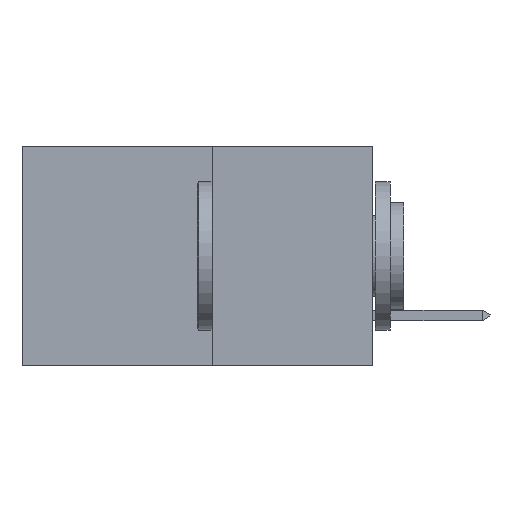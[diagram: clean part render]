
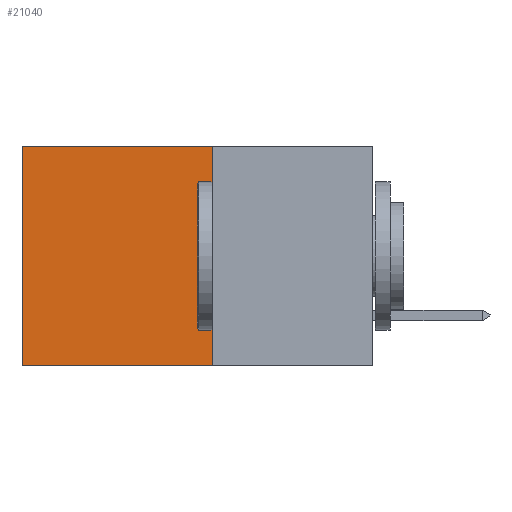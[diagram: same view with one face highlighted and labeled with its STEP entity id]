
A CAD part, left-side view. The second image highlights one B-rep face of the part: STEP entity #21040.
In plain terms, the highlighted planar face has unit normal (-1, 0, 0).
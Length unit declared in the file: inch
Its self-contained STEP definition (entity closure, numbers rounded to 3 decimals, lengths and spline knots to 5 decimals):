
#260 = DIRECTION ( 'NONE',  ( 0., 0., -1. ) ) ;
#1293 = LINE ( 'NONE', #17203, #12960 ) ;
#1573 = PLANE ( 'NONE',  #18621 ) ;
#2381 = EDGE_CURVE ( 'NONE', #3622, #14058, #3923, .T. ) ;
#2585 = CARTESIAN_POINT ( 'NONE',  ( 0.277, 0.27, 0. ) ) ;
#3622 = VERTEX_POINT ( 'NONE', #2585 ) ;
#3923 = LINE ( 'NONE', #11362, #9399 ) ;
#4416 = CARTESIAN_POINT ( 'NONE',  ( 0.277, 0.59, -0.37 ) ) ;
#6272 = DIRECTION ( 'NONE',  ( 0., 0., -1. ) ) ;
#6771 = DIRECTION ( 'NONE',  ( 0., 0., -1. ) ) ;
#6884 = CARTESIAN_POINT ( 'NONE',  ( 0.277, 0.59, 0. ) ) ;
#7058 = ORIENTED_EDGE ( 'NONE', *, *, #27936, .F. ) ;
#7704 = LINE ( 'NONE', #4416, #19350 ) ;
#9399 = VECTOR ( 'NONE', #25310, 39.37008 ) ;
#11069 = CARTESIAN_POINT ( 'NONE',  ( 0.277, 0.59, -0.37 ) ) ;
#11362 = CARTESIAN_POINT ( 'NONE',  ( 0.277, 0.27, 0. ) ) ;
#12960 = VECTOR ( 'NONE', #19562, 39.37008 ) ;
#14058 = VERTEX_POINT ( 'NONE', #6884 ) ;
#17203 = CARTESIAN_POINT ( 'NONE',  ( 0.277, 0.27, -0.37 ) ) ;
#17643 = CARTESIAN_POINT ( 'NONE',  ( 0.277, 0.27, -0.37 ) ) ;
#17770 = VERTEX_POINT ( 'NONE', #11069 ) ;
#17841 = CARTESIAN_POINT ( 'NONE',  ( 0.277, 0.27, -0.37 ) ) ;
#17953 = FACE_OUTER_BOUND ( 'NONE', #29388, .T. ) ;
#18621 = AXIS2_PLACEMENT_3D ( 'NONE', #17841, #20214, #6272 ) ;
#18826 = ORIENTED_EDGE ( 'NONE', *, *, #23870, .T. ) ;
#19350 = VECTOR ( 'NONE', #6771, 39.37008 ) ;
#19562 = DIRECTION ( 'NONE',  ( 0., 1., 0. ) ) ;
#20214 = DIRECTION ( 'NONE',  ( 1., 0., 0. ) ) ;
#20658 = VECTOR ( 'NONE', #260, 39.37008 ) ;
#20684 = ORIENTED_EDGE ( 'NONE', *, *, #27000, .F. ) ;
#21040 = ADVANCED_FACE ( 'NONE', ( #17953 ), #1573, .F. ) ;
#21368 = LINE ( 'NONE', #28152, #20658 ) ;
#23420 = ORIENTED_EDGE ( 'NONE', *, *, #2381, .T. ) ;
#23870 = EDGE_CURVE ( 'NONE', #14058, #17770, #7704, .T. ) ;
#25310 = DIRECTION ( 'NONE',  ( 0., 1., 0. ) ) ;
#27000 = EDGE_CURVE ( 'NONE', #3622, #29406, #21368, .T. ) ;
#27936 = EDGE_CURVE ( 'NONE', #29406, #17770, #1293, .T. ) ;
#28152 = CARTESIAN_POINT ( 'NONE',  ( 0.277, 0.27, -0.37 ) ) ;
#29388 = EDGE_LOOP ( 'NONE', ( #18826, #7058, #20684, #23420 ) ) ;
#29406 = VERTEX_POINT ( 'NONE', #17643 ) ;
